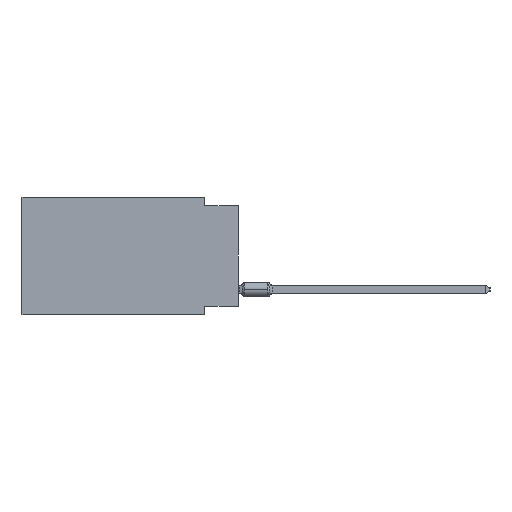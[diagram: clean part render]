
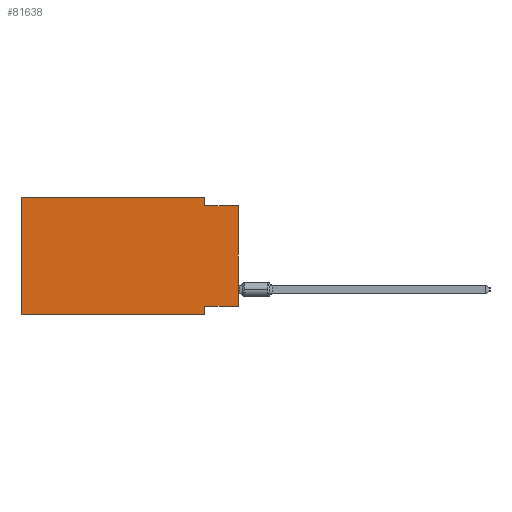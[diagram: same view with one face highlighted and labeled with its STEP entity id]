
A CAD part, left-side view. The second image highlights one B-rep face of the part: STEP entity #81638.
In plain terms, the highlighted planar face has unit normal (-1, 0, 0).
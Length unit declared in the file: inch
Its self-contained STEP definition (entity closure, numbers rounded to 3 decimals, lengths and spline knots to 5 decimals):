
#128 = VERTEX_POINT ( 'NONE', #89967 ) ;
#204 = ORIENTED_EDGE ( 'NONE', *, *, #107623, .F. ) ;
#1163 = ORIENTED_EDGE ( 'NONE', *, *, #43500, .F. ) ;
#1655 = VECTOR ( 'NONE', #28568, 39.37008 ) ;
#1918 = FACE_OUTER_BOUND ( 'NONE', #15886, .T. ) ;
#4231 = DIRECTION ( 'NONE',  ( 0., 0., -1. ) ) ;
#5352 = DIRECTION ( 'NONE',  ( 0., 1., 0. ) ) ;
#5380 = VECTOR ( 'NONE', #41493, 39.37008 ) ;
#6067 = CARTESIAN_POINT ( 'NONE',  ( 0., 0.645, 0. ) ) ;
#6215 = ORIENTED_EDGE ( 'NONE', *, *, #25152, .F. ) ;
#9543 = VECTOR ( 'NONE', #110786, 39.37008 ) ;
#9982 = VERTEX_POINT ( 'NONE', #36305 ) ;
#11535 = VERTEX_POINT ( 'NONE', #60182 ) ;
#12293 = CARTESIAN_POINT ( 'NONE',  ( 0., 0.1, 0. ) ) ;
#14002 = CARTESIAN_POINT ( 'NONE',  ( 0., 0., -0.325 ) ) ;
#15886 = EDGE_LOOP ( 'NONE', ( #49910, #89435, #34629, #6215, #1163, #60642, #204, #108006 ) ) ;
#16444 = CARTESIAN_POINT ( 'NONE',  ( 0., 0., -0.025 ) ) ;
#20283 = CARTESIAN_POINT ( 'NONE',  ( 0., 0., -0.025 ) ) ;
#21646 = CARTESIAN_POINT ( 'NONE',  ( 0., 0.645, 0. ) ) ;
#21957 = VECTOR ( 'NONE', #79819, 39.37008 ) ;
#22335 = VERTEX_POINT ( 'NONE', #58264 ) ;
#22361 = CARTESIAN_POINT ( 'NONE',  ( 0., 0.1, -0.025 ) ) ;
#25152 = EDGE_CURVE ( 'NONE', #11535, #101333, #102988, .T. ) ;
#28568 = DIRECTION ( 'NONE',  ( 0., 0., -1. ) ) ;
#34629 = ORIENTED_EDGE ( 'NONE', *, *, #57489, .F. ) ;
#35836 = CARTESIAN_POINT ( 'NONE',  ( 0., 0.645, -0.35 ) ) ;
#36305 = CARTESIAN_POINT ( 'NONE',  ( 0., 0.1, -0.35 ) ) ;
#38046 = VERTEX_POINT ( 'NONE', #22361 ) ;
#38060 = LINE ( 'NONE', #111149, #113376 ) ;
#41493 = DIRECTION ( 'NONE',  ( 0., -1., 0. ) ) ;
#41980 = EDGE_CURVE ( 'NONE', #97351, #22335, #109897, .T. ) ;
#43500 = EDGE_CURVE ( 'NONE', #128, #11535, #86803, .T. ) ;
#45119 = VERTEX_POINT ( 'NONE', #16444 ) ;
#48379 = PLANE ( 'NONE',  #73500 ) ;
#49910 = ORIENTED_EDGE ( 'NONE', *, *, #89816, .T. ) ;
#52554 = CARTESIAN_POINT ( 'NONE',  ( 0., 0.645, 0. ) ) ;
#56432 = LINE ( 'NONE', #12293, #1655 ) ;
#57416 = LINE ( 'NONE', #20283, #97033 ) ;
#57489 = EDGE_CURVE ( 'NONE', #101333, #38046, #56432, .T. ) ;
#57635 = CARTESIAN_POINT ( 'NONE',  ( 0., 0., -0.325 ) ) ;
#58264 = CARTESIAN_POINT ( 'NONE',  ( 0., 0.1, -0.325 ) ) ;
#60182 = CARTESIAN_POINT ( 'NONE',  ( 0., 0.645, 0. ) ) ;
#60642 = ORIENTED_EDGE ( 'NONE', *, *, #70193, .T. ) ;
#64443 = EDGE_CURVE ( 'NONE', #38046, #45119, #57416, .T. ) ;
#67917 = VECTOR ( 'NONE', #113644, 39.37008 ) ;
#70193 = EDGE_CURVE ( 'NONE', #128, #9982, #98484, .T. ) ;
#73500 = AXIS2_PLACEMENT_3D ( 'NONE', #21646, #90718, #4231 ) ;
#75971 = CARTESIAN_POINT ( 'NONE',  ( 0., 0.1, -0.35 ) ) ;
#76537 = LINE ( 'NONE', #75971, #9543 ) ;
#79819 = DIRECTION ( 'NONE',  ( 0., 0., 1. ) ) ;
#81638 = ADVANCED_FACE ( 'NONE', ( #1918 ), #48379, .F. ) ;
#81830 = DIRECTION ( 'NONE',  ( 0., -1., 0. ) ) ;
#86803 = LINE ( 'NONE', #52554, #21957 ) ;
#88425 = VECTOR ( 'NONE', #5352, 39.37008 ) ;
#89435 = ORIENTED_EDGE ( 'NONE', *, *, #64443, .F. ) ;
#89816 = EDGE_CURVE ( 'NONE', #97351, #45119, #38060, .T. ) ;
#89967 = CARTESIAN_POINT ( 'NONE',  ( 0., 0.645, -0.35 ) ) ;
#90718 = DIRECTION ( 'NONE',  ( 1., 0., 0. ) ) ;
#97033 = VECTOR ( 'NONE', #81830, 39.37008 ) ;
#97351 = VERTEX_POINT ( 'NONE', #14002 ) ;
#98484 = LINE ( 'NONE', #35836, #67917 ) ;
#101333 = VERTEX_POINT ( 'NONE', #111072 ) ;
#102988 = LINE ( 'NONE', #6067, #5380 ) ;
#107623 = EDGE_CURVE ( 'NONE', #22335, #9982, #76537, .T. ) ;
#108006 = ORIENTED_EDGE ( 'NONE', *, *, #41980, .F. ) ;
#108875 = DIRECTION ( 'NONE',  ( 0., 0., 1. ) ) ;
#109897 = LINE ( 'NONE', #57635, #88425 ) ;
#110786 = DIRECTION ( 'NONE',  ( 0., 0., -1. ) ) ;
#111072 = CARTESIAN_POINT ( 'NONE',  ( 0., 0.1, 0. ) ) ;
#111149 = CARTESIAN_POINT ( 'NONE',  ( 0., 0., 0. ) ) ;
#113376 = VECTOR ( 'NONE', #108875, 39.37008 ) ;
#113644 = DIRECTION ( 'NONE',  ( 0., -1., 0. ) ) ;
